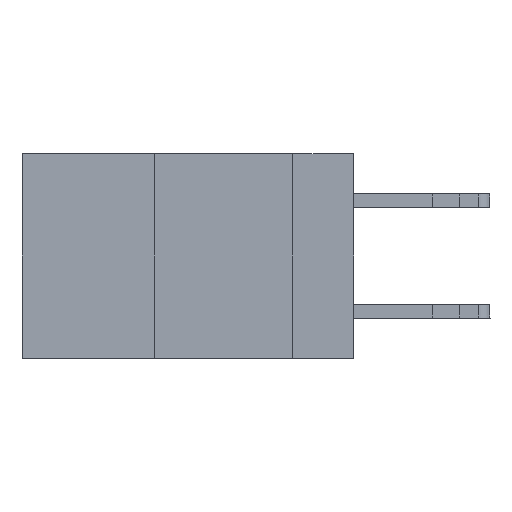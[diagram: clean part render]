
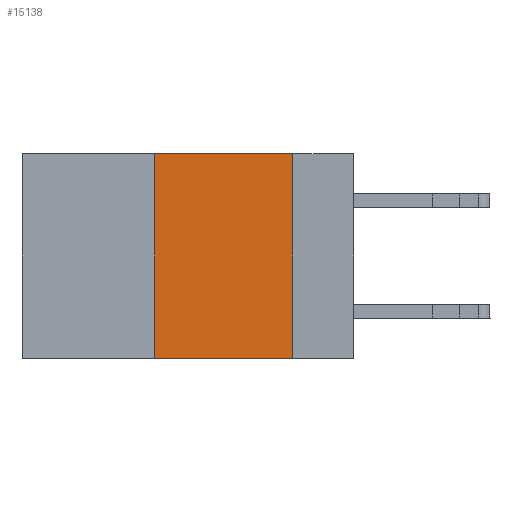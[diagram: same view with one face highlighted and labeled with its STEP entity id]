
A CAD part, left-side view. The second image highlights one B-rep face of the part: STEP entity #15138.
In plain terms, the highlighted planar face has unit normal (-1, 0, 0).
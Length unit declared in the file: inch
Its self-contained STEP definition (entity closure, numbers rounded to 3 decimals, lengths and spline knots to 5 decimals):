
#1705 = LINE ( 'NONE', #9976, #19418 ) ;
#2417 = VERTEX_POINT ( 'NONE', #7703 ) ;
#2957 = LINE ( 'NONE', #14029, #9798 ) ;
#3168 = CARTESIAN_POINT ( 'NONE',  ( 0., 0.6, 0. ) ) ;
#3265 = DIRECTION ( 'NONE',  ( 0., -1., 0. ) ) ;
#3627 = DIRECTION ( 'NONE',  ( 0., 0., -1. ) ) ;
#4799 = VERTEX_POINT ( 'NONE', #16828 ) ;
#5069 = DIRECTION ( 'NONE',  ( 0., 0., 1. ) ) ;
#5506 = LINE ( 'NONE', #5604, #17527 ) ;
#5604 = CARTESIAN_POINT ( 'NONE',  ( 0., 0.11, 0. ) ) ;
#5878 = EDGE_CURVE ( 'NONE', #15117, #2417, #2957, .T. ) ;
#6283 = CARTESIAN_POINT ( 'NONE',  ( 0., 0.36, 0. ) ) ;
#6503 = PLANE ( 'NONE',  #18117 ) ;
#6598 = FACE_OUTER_BOUND ( 'NONE', #17843, .T. ) ;
#7703 = CARTESIAN_POINT ( 'NONE',  ( 0., 0.11, 0. ) ) ;
#9798 = VECTOR ( 'NONE', #13830, 39.37008 ) ;
#9853 = CARTESIAN_POINT ( 'NONE',  ( 0., 0.6, -0.37 ) ) ;
#9976 = CARTESIAN_POINT ( 'NONE',  ( 0., 0.36, 0. ) ) ;
#11669 = ORIENTED_EDGE ( 'NONE', *, *, #14816, .F. ) ;
#12982 = DIRECTION ( 'NONE',  ( 0., 0., -1. ) ) ;
#13830 = DIRECTION ( 'NONE',  ( 0., -1., 0. ) ) ;
#14029 = CARTESIAN_POINT ( 'NONE',  ( 0., 0.6, 0. ) ) ;
#14114 = VERTEX_POINT ( 'NONE', #18884 ) ;
#14816 = EDGE_CURVE ( 'NONE', #4799, #15117, #1705, .T. ) ;
#15117 = VERTEX_POINT ( 'NONE', #6283 ) ;
#15130 = EDGE_CURVE ( 'NONE', #4799, #14114, #18733, .T. ) ;
#15138 = ADVANCED_FACE ( 'NONE', ( #6598 ), #6503, .F. ) ;
#15911 = DIRECTION ( 'NONE',  ( 1., 0., 0. ) ) ;
#16117 = VECTOR ( 'NONE', #3265, 39.37008 ) ;
#16529 = ORIENTED_EDGE ( 'NONE', *, *, #15130, .T. ) ;
#16828 = CARTESIAN_POINT ( 'NONE',  ( 0., 0.36, -0.37 ) ) ;
#17081 = ORIENTED_EDGE ( 'NONE', *, *, #18369, .F. ) ;
#17527 = VECTOR ( 'NONE', #3627, 39.37008 ) ;
#17843 = EDGE_LOOP ( 'NONE', ( #17081, #20662, #11669, #16529 ) ) ;
#18117 = AXIS2_PLACEMENT_3D ( 'NONE', #3168, #15911, #12982 ) ;
#18369 = EDGE_CURVE ( 'NONE', #2417, #14114, #5506, .T. ) ;
#18733 = LINE ( 'NONE', #9853, #16117 ) ;
#18884 = CARTESIAN_POINT ( 'NONE',  ( 0., 0.11, -0.37 ) ) ;
#19418 = VECTOR ( 'NONE', #5069, 39.37008 ) ;
#20662 = ORIENTED_EDGE ( 'NONE', *, *, #5878, .F. ) ;
